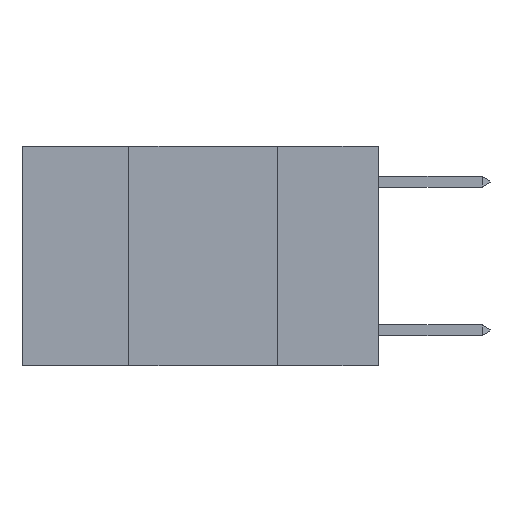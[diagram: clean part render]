
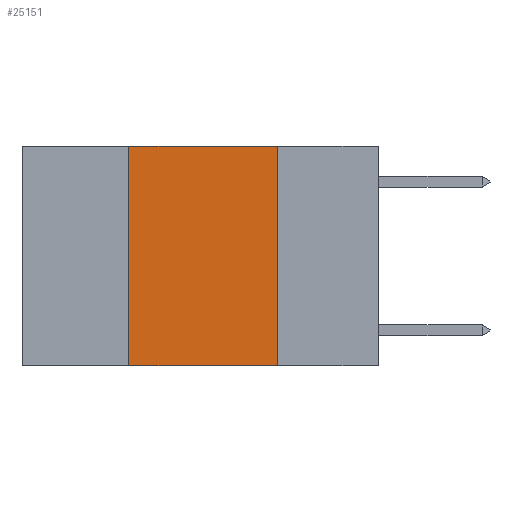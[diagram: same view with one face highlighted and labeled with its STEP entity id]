
A CAD part, left-side view. The second image highlights one B-rep face of the part: STEP entity #25151.
In plain terms, the highlighted planar face has unit normal (-1, 0, 0).
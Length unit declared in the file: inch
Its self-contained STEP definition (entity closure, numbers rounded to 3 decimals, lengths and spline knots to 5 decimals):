
#87 = VERTEX_POINT ( 'NONE', #205 ) ;
#163 = PLANE ( 'NONE',  #12078 ) ;
#205 = CARTESIAN_POINT ( 'NONE',  ( 0., 0.17, -0.37 ) ) ;
#1109 = LINE ( 'NONE', #6300, #28533 ) ;
#4195 = CARTESIAN_POINT ( 'NONE',  ( 0., 0.17, 0. ) ) ;
#5040 = DIRECTION ( 'NONE',  ( 0., -1., 0. ) ) ;
#6300 = CARTESIAN_POINT ( 'NONE',  ( 0., 0.42, 0. ) ) ;
#6881 = DIRECTION ( 'NONE',  ( 0., 0., -1. ) ) ;
#6912 = LINE ( 'NONE', #26414, #12784 ) ;
#8179 = LINE ( 'NONE', #22378, #25215 ) ;
#8520 = DIRECTION ( 'NONE',  ( 0., 0., 1. ) ) ;
#9786 = EDGE_CURVE ( 'NONE', #20133, #87, #6912, .T. ) ;
#10482 = CARTESIAN_POINT ( 'NONE',  ( 0., 0.42, 0. ) ) ;
#12078 = AXIS2_PLACEMENT_3D ( 'NONE', #13436, #20125, #6881 ) ;
#12784 = VECTOR ( 'NONE', #28616, 39.37008 ) ;
#13436 = CARTESIAN_POINT ( 'NONE',  ( 0., 0.6, 0. ) ) ;
#14548 = ORIENTED_EDGE ( 'NONE', *, *, #23181, .F. ) ;
#14567 = ORIENTED_EDGE ( 'NONE', *, *, #21320, .F. ) ;
#14929 = ORIENTED_EDGE ( 'NONE', *, *, #18663, .F. ) ;
#15014 = ORIENTED_EDGE ( 'NONE', *, *, #9786, .T. ) ;
#17255 = FACE_OUTER_BOUND ( 'NONE', #27463, .T. ) ;
#18018 = VERTEX_POINT ( 'NONE', #10482 ) ;
#18657 = VECTOR ( 'NONE', #5040, 39.37008 ) ;
#18663 = EDGE_CURVE ( 'NONE', #20133, #18018, #1109, .T. ) ;
#19004 = CARTESIAN_POINT ( 'NONE',  ( 0., 0.42, -0.37 ) ) ;
#20125 = DIRECTION ( 'NONE',  ( 1., 0., 0. ) ) ;
#20133 = VERTEX_POINT ( 'NONE', #19004 ) ;
#21320 = EDGE_CURVE ( 'NONE', #18018, #25896, #25316, .T. ) ;
#22378 = CARTESIAN_POINT ( 'NONE',  ( 0., 0.17, 0. ) ) ;
#22681 = CARTESIAN_POINT ( 'NONE',  ( 0., 0.6, 0. ) ) ;
#23181 = EDGE_CURVE ( 'NONE', #25896, #87, #8179, .T. ) ;
#24638 = DIRECTION ( 'NONE',  ( 0., 0., -1. ) ) ;
#25151 = ADVANCED_FACE ( 'NONE', ( #17255 ), #163, .F. ) ;
#25215 = VECTOR ( 'NONE', #24638, 39.37008 ) ;
#25316 = LINE ( 'NONE', #22681, #18657 ) ;
#25896 = VERTEX_POINT ( 'NONE', #4195 ) ;
#26414 = CARTESIAN_POINT ( 'NONE',  ( 0., 0.6, -0.37 ) ) ;
#27463 = EDGE_LOOP ( 'NONE', ( #14548, #14567, #14929, #15014 ) ) ;
#28533 = VECTOR ( 'NONE', #8520, 39.37008 ) ;
#28616 = DIRECTION ( 'NONE',  ( 0., -1., 0. ) ) ;
